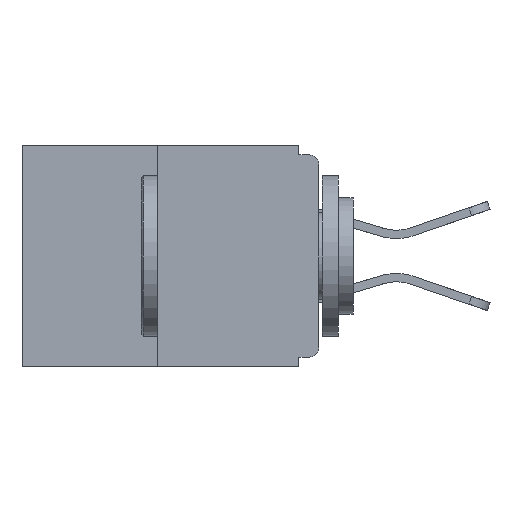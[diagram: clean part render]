
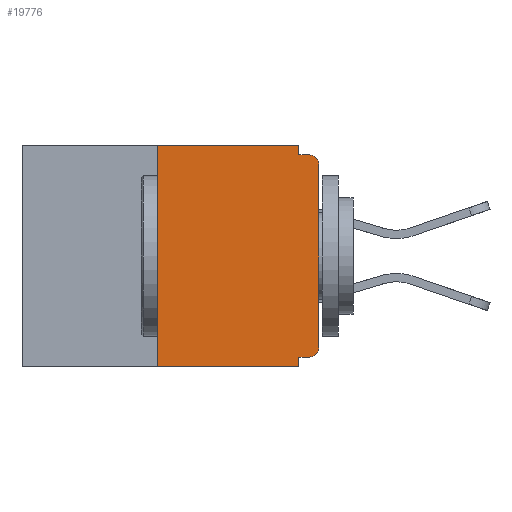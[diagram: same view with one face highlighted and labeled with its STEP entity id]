
A CAD part, left-side view. The second image highlights one B-rep face of the part: STEP entity #19776.
In plain terms, the highlighted planar face has unit normal (-1, 0, 0).
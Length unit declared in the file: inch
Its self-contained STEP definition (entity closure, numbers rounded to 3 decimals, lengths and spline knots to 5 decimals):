
#54 = VERTEX_POINT ( 'NONE', #24782 ) ;
#585 = DIRECTION ( 'NONE',  ( 0., 0., -1. ) ) ;
#1533 = LINE ( 'NONE', #25031, #18038 ) ;
#2768 = VECTOR ( 'NONE', #24442, 39.37008 ) ;
#3486 = EDGE_CURVE ( 'NONE', #21274, #25754, #26038, .T. ) ;
#3641 = EDGE_CURVE ( 'NONE', #54, #12818, #6383, .T. ) ;
#3650 = CARTESIAN_POINT ( 'NONE',  ( 0., 0.031, -0.328 ) ) ;
#3790 = CIRCLE ( 'NONE', #17486, 0.015 ) ;
#4215 = CARTESIAN_POINT ( 'NONE',  ( 0., 0.031, -0.015 ) ) ;
#4493 = VERTEX_POINT ( 'NONE', #4215 ) ;
#5212 = DIRECTION ( 'NONE',  ( 0., -1., 0. ) ) ;
#5300 = DIRECTION ( 'NONE',  ( 1., 0., 0. ) ) ;
#5312 = CARTESIAN_POINT ( 'NONE',  ( 0., 0., -0.313 ) ) ;
#5514 = DIRECTION ( 'NONE',  ( 0., 0., -1. ) ) ;
#5555 = ORIENTED_EDGE ( 'NONE', *, *, #19766, .F. ) ;
#6031 = ORIENTED_EDGE ( 'NONE', *, *, #15923, .T. ) ;
#6157 = DIRECTION ( 'NONE',  ( 0., 0., -1. ) ) ;
#6383 = LINE ( 'NONE', #30686, #26004 ) ;
#7187 = CARTESIAN_POINT ( 'NONE',  ( 0., 0., -0.015 ) ) ;
#7677 = DIRECTION ( 'NONE',  ( -1., 0., 0. ) ) ;
#7781 = DIRECTION ( 'NONE',  ( 0., 0., -1. ) ) ;
#7953 = CARTESIAN_POINT ( 'NONE',  ( 0., 0.031, 0. ) ) ;
#7970 = PLANE ( 'NONE',  #23051 ) ;
#8104 = VERTEX_POINT ( 'NONE', #21773 ) ;
#8259 = LINE ( 'NONE', #20034, #17091 ) ;
#8342 = CARTESIAN_POINT ( 'NONE',  ( 0., 0.46, 0. ) ) ;
#9398 = CARTESIAN_POINT ( 'NONE',  ( 0., 0.015, -0.015 ) ) ;
#9688 = ORIENTED_EDGE ( 'NONE', *, *, #30967, .T. ) ;
#9948 = LINE ( 'NONE', #28657, #19171 ) ;
#10610 = LINE ( 'NONE', #17644, #19022 ) ;
#11419 = EDGE_LOOP ( 'NONE', ( #25860, #5555, #6031, #12461, #29987, #19989, #9688, #13312, #22721, #18163 ) ) ;
#11427 = EDGE_CURVE ( 'NONE', #4493, #29141, #21622, .T. ) ;
#11732 = FACE_OUTER_BOUND ( 'NONE', #11419, .T. ) ;
#11771 = AXIS2_PLACEMENT_3D ( 'NONE', #17884, #7677, #7781 ) ;
#12382 = EDGE_CURVE ( 'NONE', #25754, #4493, #9948, .T. ) ;
#12461 = ORIENTED_EDGE ( 'NONE', *, *, #19758, .F. ) ;
#12818 = VERTEX_POINT ( 'NONE', #3650 ) ;
#13312 = ORIENTED_EDGE ( 'NONE', *, *, #26218, .T. ) ;
#13583 = VERTEX_POINT ( 'NONE', #27796 ) ;
#15254 = VECTOR ( 'NONE', #16375, 39.37008 ) ;
#15388 = VERTEX_POINT ( 'NONE', #5312 ) ;
#15923 = EDGE_CURVE ( 'NONE', #13583, #18092, #20383, .T. ) ;
#16375 = DIRECTION ( 'NONE',  ( 0., -1., 0. ) ) ;
#16691 = CARTESIAN_POINT ( 'NONE',  ( 0., 0.031, -0.343 ) ) ;
#17091 = VECTOR ( 'NONE', #29828, 39.37008 ) ;
#17486 = AXIS2_PLACEMENT_3D ( 'NONE', #30174, #18704, #6157 ) ;
#17644 = CARTESIAN_POINT ( 'NONE',  ( 0., 0.031, -0.343 ) ) ;
#17884 = CARTESIAN_POINT ( 'NONE',  ( 0., 0.015, -0.313 ) ) ;
#18038 = VECTOR ( 'NONE', #18190, 39.37008 ) ;
#18092 = VERTEX_POINT ( 'NONE', #16691 ) ;
#18163 = ORIENTED_EDGE ( 'NONE', *, *, #12382, .F. ) ;
#18190 = DIRECTION ( 'NONE',  ( 0., 0., 1. ) ) ;
#18443 = CARTESIAN_POINT ( 'NONE',  ( 0., 0.25, 0. ) ) ;
#18704 = DIRECTION ( 'NONE',  ( -1., 0., 0. ) ) ;
#19022 = VECTOR ( 'NONE', #585, 39.37008 ) ;
#19171 = VECTOR ( 'NONE', #21235, 39.37008 ) ;
#19758 = EDGE_CURVE ( 'NONE', #12818, #18092, #10610, .T. ) ;
#19766 = EDGE_CURVE ( 'NONE', #13583, #21274, #8259, .T. ) ;
#19776 = ADVANCED_FACE ( 'NONE', ( #11732 ), #7970, .F. ) ;
#19989 = ORIENTED_EDGE ( 'NONE', *, *, #23182, .T. ) ;
#20034 = CARTESIAN_POINT ( 'NONE',  ( 0., 0.25, 0. ) ) ;
#20383 = LINE ( 'NONE', #20509, #29612 ) ;
#20509 = CARTESIAN_POINT ( 'NONE',  ( 0., 0.46, -0.343 ) ) ;
#21235 = DIRECTION ( 'NONE',  ( 0., 0., -1. ) ) ;
#21274 = VERTEX_POINT ( 'NONE', #18443 ) ;
#21622 = LINE ( 'NONE', #7187, #2768 ) ;
#21773 = CARTESIAN_POINT ( 'NONE',  ( 0., 0., -0.03 ) ) ;
#22721 = ORIENTED_EDGE ( 'NONE', *, *, #11427, .F. ) ;
#23051 = AXIS2_PLACEMENT_3D ( 'NONE', #30037, #5300, #5514 ) ;
#23182 = EDGE_CURVE ( 'NONE', #54, #15388, #30896, .T. ) ;
#24442 = DIRECTION ( 'NONE',  ( 0., -1., 0. ) ) ;
#24782 = CARTESIAN_POINT ( 'NONE',  ( 0., 0.015, -0.328 ) ) ;
#25031 = CARTESIAN_POINT ( 'NONE',  ( 0., 0., 0. ) ) ;
#25754 = VERTEX_POINT ( 'NONE', #7953 ) ;
#25860 = ORIENTED_EDGE ( 'NONE', *, *, #3486, .F. ) ;
#26004 = VECTOR ( 'NONE', #26075, 39.37008 ) ;
#26038 = LINE ( 'NONE', #8342, #15254 ) ;
#26075 = DIRECTION ( 'NONE',  ( 0., 1., 0. ) ) ;
#26218 = EDGE_CURVE ( 'NONE', #8104, #29141, #3790, .T. ) ;
#27796 = CARTESIAN_POINT ( 'NONE',  ( 0., 0.25, -0.343 ) ) ;
#28657 = CARTESIAN_POINT ( 'NONE',  ( 0., 0.031, 0. ) ) ;
#29141 = VERTEX_POINT ( 'NONE', #9398 ) ;
#29612 = VECTOR ( 'NONE', #5212, 39.37008 ) ;
#29828 = DIRECTION ( 'NONE',  ( 0., 0., 1. ) ) ;
#29987 = ORIENTED_EDGE ( 'NONE', *, *, #3641, .F. ) ;
#30037 = CARTESIAN_POINT ( 'NONE',  ( 0., 0.46, 0. ) ) ;
#30174 = CARTESIAN_POINT ( 'NONE',  ( 0., 0.015, -0.03 ) ) ;
#30686 = CARTESIAN_POINT ( 'NONE',  ( 0., 0., -0.328 ) ) ;
#30896 = CIRCLE ( 'NONE', #11771, 0.015 ) ;
#30967 = EDGE_CURVE ( 'NONE', #15388, #8104, #1533, .T. ) ;
